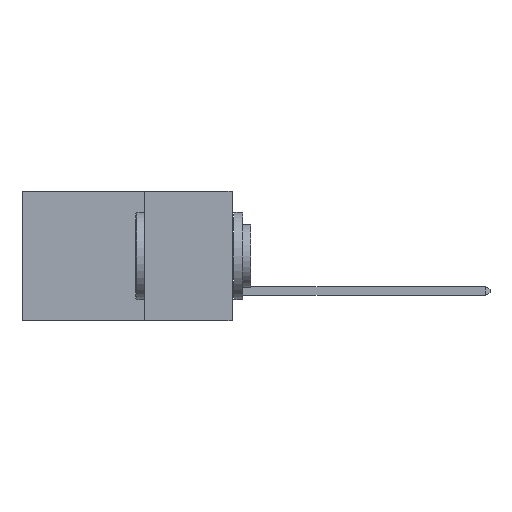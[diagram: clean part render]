
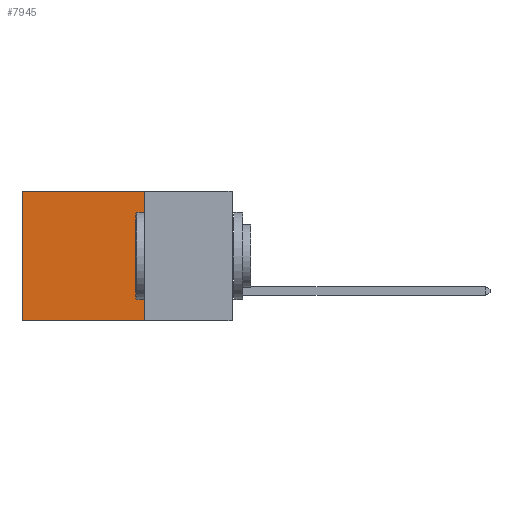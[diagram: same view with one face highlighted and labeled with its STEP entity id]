
A CAD part, left-side view. The second image highlights one B-rep face of the part: STEP entity #7945.
In plain terms, the highlighted planar face has unit normal (-1, 0, 0).
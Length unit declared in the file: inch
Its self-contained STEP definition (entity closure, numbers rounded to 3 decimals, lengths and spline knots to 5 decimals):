
#49 = CARTESIAN_POINT ( 'NONE',  ( 0.2875, 0.6, 0. ) ) ;
#56 = CARTESIAN_POINT ( 'NONE',  ( 0.2875, 0.25, 0. ) ) ;
#312 = EDGE_CURVE ( 'NONE', #1668, #17467, #15618, .T. ) ;
#1048 = DIRECTION ( 'NONE',  ( 0., 1., 0. ) ) ;
#1295 = EDGE_LOOP ( 'NONE', ( #20675, #7832, #6710, #16965 ) ) ;
#1668 = VERTEX_POINT ( 'NONE', #11110 ) ;
#2173 = EDGE_CURVE ( 'NONE', #18636, #1668, #15810, .T. ) ;
#2337 = VECTOR ( 'NONE', #1048, 39.37008 ) ;
#3095 = CARTESIAN_POINT ( 'NONE',  ( 0.2875, 0.25, 0. ) ) ;
#4216 = DIRECTION ( 'NONE',  ( 0., 0., -1. ) ) ;
#5185 = CARTESIAN_POINT ( 'NONE',  ( 0.2875, 0.25, -0.37 ) ) ;
#6004 = CARTESIAN_POINT ( 'NONE',  ( 0.2875, 0.25, 0. ) ) ;
#6710 = ORIENTED_EDGE ( 'NONE', *, *, #12067, .F. ) ;
#7123 = LINE ( 'NONE', #56, #12073 ) ;
#7721 = DIRECTION ( 'NONE',  ( 0., 0., -1. ) ) ;
#7832 = ORIENTED_EDGE ( 'NONE', *, *, #19235, .F. ) ;
#7945 = ADVANCED_FACE ( 'NONE', ( #15837 ), #14367, .F. ) ;
#8102 = VECTOR ( 'NONE', #21367, 39.37008 ) ;
#11110 = CARTESIAN_POINT ( 'NONE',  ( 0.2875, 0.6, 0. ) ) ;
#12067 = EDGE_CURVE ( 'NONE', #18636, #13539, #7123, .T. ) ;
#12073 = VECTOR ( 'NONE', #12103, 39.37008 ) ;
#12103 = DIRECTION ( 'NONE',  ( 0., 0., -1. ) ) ;
#12550 = LINE ( 'NONE', #14909, #8102 ) ;
#13539 = VERTEX_POINT ( 'NONE', #5185 ) ;
#14367 = PLANE ( 'NONE',  #20256 ) ;
#14909 = CARTESIAN_POINT ( 'NONE',  ( 0.2875, 0.25, -0.37 ) ) ;
#15618 = LINE ( 'NONE', #49, #17906 ) ;
#15810 = LINE ( 'NONE', #3095, #2337 ) ;
#15837 = FACE_OUTER_BOUND ( 'NONE', #1295, .T. ) ;
#16965 = ORIENTED_EDGE ( 'NONE', *, *, #2173, .T. ) ;
#17467 = VERTEX_POINT ( 'NONE', #17900 ) ;
#17646 = DIRECTION ( 'NONE',  ( 1., 0., 0. ) ) ;
#17900 = CARTESIAN_POINT ( 'NONE',  ( 0.2875, 0.6, -0.37 ) ) ;
#17906 = VECTOR ( 'NONE', #4216, 39.37008 ) ;
#18636 = VERTEX_POINT ( 'NONE', #21396 ) ;
#19235 = EDGE_CURVE ( 'NONE', #13539, #17467, #12550, .T. ) ;
#20256 = AXIS2_PLACEMENT_3D ( 'NONE', #6004, #17646, #7721 ) ;
#20675 = ORIENTED_EDGE ( 'NONE', *, *, #312, .T. ) ;
#21367 = DIRECTION ( 'NONE',  ( 0., 1., 0. ) ) ;
#21396 = CARTESIAN_POINT ( 'NONE',  ( 0.2875, 0.25, 0. ) ) ;
